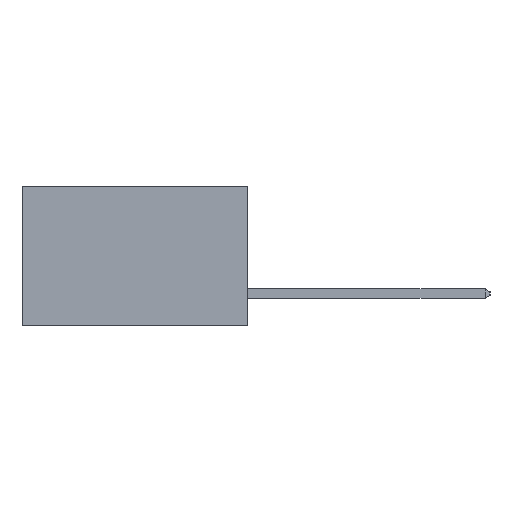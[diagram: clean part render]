
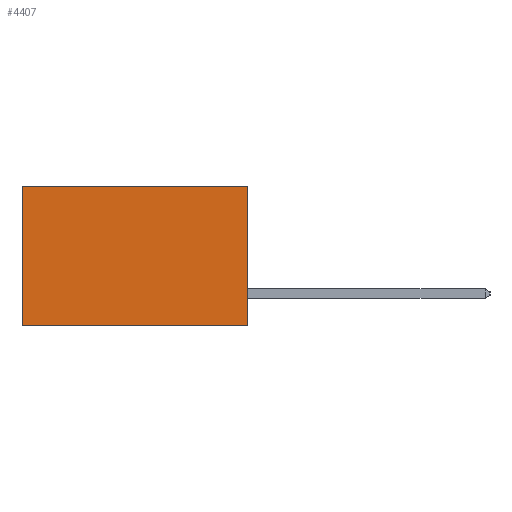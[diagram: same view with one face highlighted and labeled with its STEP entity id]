
A CAD part, left-side view. The second image highlights one B-rep face of the part: STEP entity #4407.
In plain terms, the highlighted planar face has unit normal (-1, 0, 0).
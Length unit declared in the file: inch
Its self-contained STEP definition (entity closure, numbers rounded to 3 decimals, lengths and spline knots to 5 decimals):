
#390 = ORIENTED_EDGE ( 'NONE', *, *, #9982, .T. ) ;
#1372 = ORIENTED_EDGE ( 'NONE', *, *, #2902, .F. ) ;
#2902 = EDGE_CURVE ( 'NONE', #3220, #9630, #15762, .T. ) ;
#3220 = VERTEX_POINT ( 'NONE', #6812 ) ;
#3979 = EDGE_LOOP ( 'NONE', ( #7429, #14832, #1372, #390 ) ) ;
#4407 = ADVANCED_FACE ( 'NONE', ( #15987 ), #22733, .F. ) ;
#5720 = CARTESIAN_POINT ( 'NONE',  ( 0.2615, 0., 0. ) ) ;
#5904 = DIRECTION ( 'NONE',  ( 0., 1., 0. ) ) ;
#5956 = CARTESIAN_POINT ( 'NONE',  ( 0.2615, 0.6, -0.37 ) ) ;
#6573 = AXIS2_PLACEMENT_3D ( 'NONE', #24711, #14779, #14840 ) ;
#6812 = CARTESIAN_POINT ( 'NONE',  ( 0.2615, 0., 0. ) ) ;
#7396 = CARTESIAN_POINT ( 'NONE',  ( 0.2615, 0.6, 0. ) ) ;
#7429 = ORIENTED_EDGE ( 'NONE', *, *, #12439, .T. ) ;
#9630 = VERTEX_POINT ( 'NONE', #16929 ) ;
#9780 = VECTOR ( 'NONE', #14757, 39.37008 ) ;
#9982 = EDGE_CURVE ( 'NONE', #3220, #13548, #13867, .T. ) ;
#11347 = CARTESIAN_POINT ( 'NONE',  ( 0.2615, 0.6, -0.37 ) ) ;
#12439 = EDGE_CURVE ( 'NONE', #13548, #16078, #20833, .T. ) ;
#12861 = VECTOR ( 'NONE', #19622, 39.37008 ) ;
#13548 = VERTEX_POINT ( 'NONE', #7396 ) ;
#13867 = LINE ( 'NONE', #5720, #23098 ) ;
#14757 = DIRECTION ( 'NONE',  ( 0., 0., -1. ) ) ;
#14779 = DIRECTION ( 'NONE',  ( 1., 0., 0. ) ) ;
#14832 = ORIENTED_EDGE ( 'NONE', *, *, #22559, .F. ) ;
#14840 = DIRECTION ( 'NONE',  ( 0., 0., -1. ) ) ;
#14850 = CARTESIAN_POINT ( 'NONE',  ( 0.2615, 0., -0.37 ) ) ;
#15762 = LINE ( 'NONE', #14850, #9780 ) ;
#15987 = FACE_OUTER_BOUND ( 'NONE', #3979, .T. ) ;
#16078 = VERTEX_POINT ( 'NONE', #11347 ) ;
#16929 = CARTESIAN_POINT ( 'NONE',  ( 0.2615, 0., -0.37 ) ) ;
#17650 = CARTESIAN_POINT ( 'NONE',  ( 0.2615, 0., -0.37 ) ) ;
#19622 = DIRECTION ( 'NONE',  ( 0., 1., 0. ) ) ;
#20833 = LINE ( 'NONE', #5956, #25364 ) ;
#21873 = DIRECTION ( 'NONE',  ( 0., 0., -1. ) ) ;
#22559 = EDGE_CURVE ( 'NONE', #9630, #16078, #23347, .T. ) ;
#22733 = PLANE ( 'NONE',  #6573 ) ;
#23098 = VECTOR ( 'NONE', #5904, 39.37008 ) ;
#23347 = LINE ( 'NONE', #17650, #12861 ) ;
#24711 = CARTESIAN_POINT ( 'NONE',  ( 0.2615, 0., -0.37 ) ) ;
#25364 = VECTOR ( 'NONE', #21873, 39.37008 ) ;
